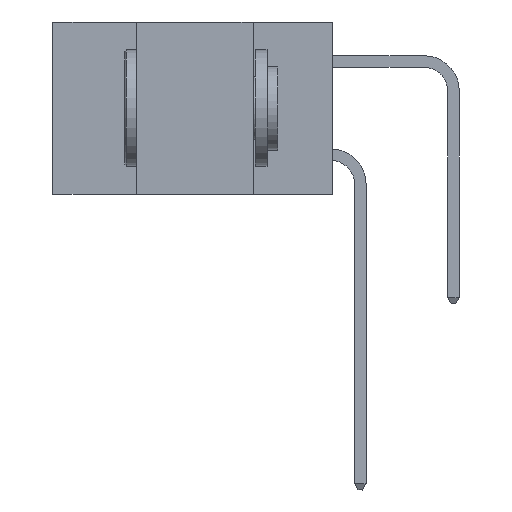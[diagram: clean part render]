
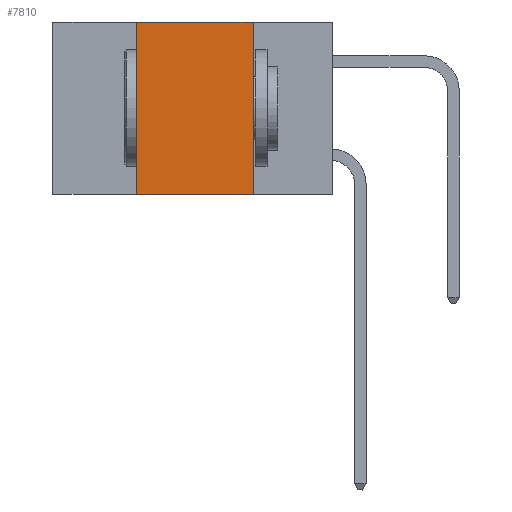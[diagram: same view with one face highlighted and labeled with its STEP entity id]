
A CAD part, left-side view. The second image highlights one B-rep face of the part: STEP entity #7810.
In plain terms, the highlighted planar face has unit normal (-1, 0, 0).
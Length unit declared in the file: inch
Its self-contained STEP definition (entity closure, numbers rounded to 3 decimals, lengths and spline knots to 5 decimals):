
#590 = EDGE_CURVE ( 'NONE', #2244, #2796, #4786, .T. ) ;
#1306 = CARTESIAN_POINT ( 'NONE',  ( 0., 0.6, -0.37 ) ) ;
#2244 = VERTEX_POINT ( 'NONE', #7203 ) ;
#2419 = ORIENTED_EDGE ( 'NONE', *, *, #590, .F. ) ;
#2796 = VERTEX_POINT ( 'NONE', #9441 ) ;
#3475 = DIRECTION ( 'NONE',  ( 0., -1., 0. ) ) ;
#4082 = DIRECTION ( 'NONE',  ( 0., -1., 0. ) ) ;
#4628 = PLANE ( 'NONE',  #5740 ) ;
#4786 = LINE ( 'NONE', #11752, #13364 ) ;
#5588 = DIRECTION ( 'NONE',  ( 1., 0., 0. ) ) ;
#5740 = AXIS2_PLACEMENT_3D ( 'NONE', #13395, #5588, #10119 ) ;
#5924 = VECTOR ( 'NONE', #4082, 39.37008 ) ;
#6110 = EDGE_LOOP ( 'NONE', ( #14117, #10861, #2419, #6503 ) ) ;
#6503 = ORIENTED_EDGE ( 'NONE', *, *, #10068, .T. ) ;
#6895 = EDGE_CURVE ( 'NONE', #12877, #9004, #9386, .T. ) ;
#7203 = CARTESIAN_POINT ( 'NONE',  ( 0., 0.42, -0.37 ) ) ;
#7387 = DIRECTION ( 'NONE',  ( 0., 0., 1. ) ) ;
#7810 = ADVANCED_FACE ( 'NONE', ( #14086 ), #4628, .F. ) ;
#8567 = CARTESIAN_POINT ( 'NONE',  ( 0., 0.6, 0. ) ) ;
#9004 = VERTEX_POINT ( 'NONE', #10559 ) ;
#9386 = LINE ( 'NONE', #11017, #12681 ) ;
#9441 = CARTESIAN_POINT ( 'NONE',  ( 0., 0.42, 0. ) ) ;
#9493 = LINE ( 'NONE', #1306, #11420 ) ;
#10068 = EDGE_CURVE ( 'NONE', #2244, #9004, #9493, .T. ) ;
#10119 = DIRECTION ( 'NONE',  ( 0., 0., -1. ) ) ;
#10477 = EDGE_CURVE ( 'NONE', #2796, #12877, #13858, .T. ) ;
#10559 = CARTESIAN_POINT ( 'NONE',  ( 0., 0.17, -0.37 ) ) ;
#10861 = ORIENTED_EDGE ( 'NONE', *, *, #10477, .F. ) ;
#11017 = CARTESIAN_POINT ( 'NONE',  ( 0., 0.17, 0. ) ) ;
#11420 = VECTOR ( 'NONE', #3475, 39.37008 ) ;
#11752 = CARTESIAN_POINT ( 'NONE',  ( 0., 0.42, 0. ) ) ;
#12210 = DIRECTION ( 'NONE',  ( 0., 0., -1. ) ) ;
#12681 = VECTOR ( 'NONE', #12210, 39.37008 ) ;
#12877 = VERTEX_POINT ( 'NONE', #14422 ) ;
#13364 = VECTOR ( 'NONE', #7387, 39.37008 ) ;
#13395 = CARTESIAN_POINT ( 'NONE',  ( 0., 0.6, 0. ) ) ;
#13858 = LINE ( 'NONE', #8567, #5924 ) ;
#14086 = FACE_OUTER_BOUND ( 'NONE', #6110, .T. ) ;
#14117 = ORIENTED_EDGE ( 'NONE', *, *, #6895, .F. ) ;
#14422 = CARTESIAN_POINT ( 'NONE',  ( 0., 0.17, 0. ) ) ;
